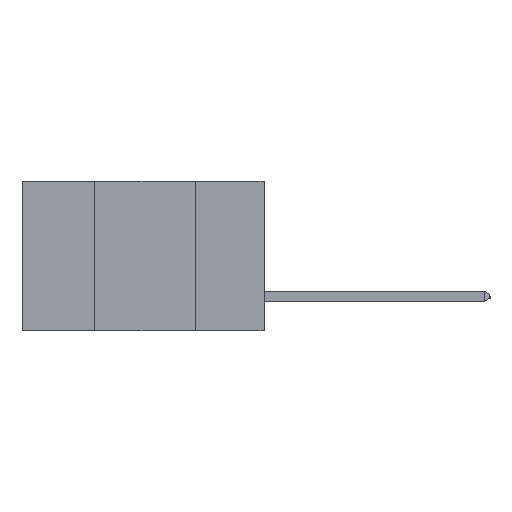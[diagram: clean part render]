
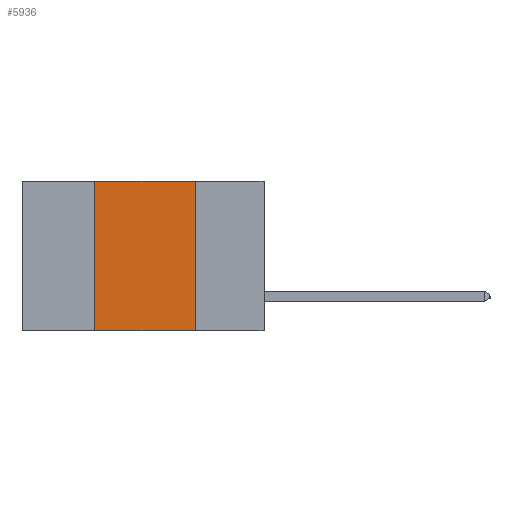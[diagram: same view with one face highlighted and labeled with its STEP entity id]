
A CAD part, left-side view. The second image highlights one B-rep face of the part: STEP entity #5936.
In plain terms, the highlighted planar face has unit normal (-1, 0, 0).
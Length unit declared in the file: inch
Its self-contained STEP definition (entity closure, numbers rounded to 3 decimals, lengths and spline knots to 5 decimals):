
#427 = CARTESIAN_POINT ( 'NONE',  ( 0., 0.42, -0.37 ) ) ;
#438 = VECTOR ( 'NONE', #7719, 39.37008 ) ;
#1325 = CARTESIAN_POINT ( 'NONE',  ( 0., 0.6, 0. ) ) ;
#1400 = ORIENTED_EDGE ( 'NONE', *, *, #5030, .F. ) ;
#1433 = ORIENTED_EDGE ( 'NONE', *, *, #4392, .F. ) ;
#1859 = FACE_OUTER_BOUND ( 'NONE', #6535, .T. ) ;
#2053 = VERTEX_POINT ( 'NONE', #9306 ) ;
#2086 = ORIENTED_EDGE ( 'NONE', *, *, #10315, .T. ) ;
#2499 = CARTESIAN_POINT ( 'NONE',  ( 0., 0.6, 0. ) ) ;
#3251 = DIRECTION ( 'NONE',  ( 0., 0., 1. ) ) ;
#3254 = CARTESIAN_POINT ( 'NONE',  ( 0., 0.42, 0. ) ) ;
#3283 = EDGE_CURVE ( 'NONE', #7934, #3319, #8841, .T. ) ;
#3319 = VERTEX_POINT ( 'NONE', #8916 ) ;
#3467 = DIRECTION ( 'NONE',  ( 1., 0., 0. ) ) ;
#4392 = EDGE_CURVE ( 'NONE', #2053, #7729, #8712, .T. ) ;
#4463 = CARTESIAN_POINT ( 'NONE',  ( 0., 0.17, -0.37 ) ) ;
#4879 = VECTOR ( 'NONE', #3251, 39.37008 ) ;
#5030 = EDGE_CURVE ( 'NONE', #3319, #2053, #8929, .T. ) ;
#5333 = PLANE ( 'NONE',  #9651 ) ;
#5475 = CARTESIAN_POINT ( 'NONE',  ( 0., 0.6, -0.37 ) ) ;
#5936 = ADVANCED_FACE ( 'NONE', ( #1859 ), #5333, .F. ) ;
#6320 = DIRECTION ( 'NONE',  ( 0., -1., 0. ) ) ;
#6535 = EDGE_LOOP ( 'NONE', ( #1433, #1400, #8598, #2086 ) ) ;
#7719 = DIRECTION ( 'NONE',  ( 0., -1., 0. ) ) ;
#7729 = VERTEX_POINT ( 'NONE', #4463 ) ;
#7934 = VERTEX_POINT ( 'NONE', #427 ) ;
#8313 = LINE ( 'NONE', #5475, #10016 ) ;
#8598 = ORIENTED_EDGE ( 'NONE', *, *, #3283, .F. ) ;
#8712 = LINE ( 'NONE', #10352, #10399 ) ;
#8841 = LINE ( 'NONE', #3254, #4879 ) ;
#8916 = CARTESIAN_POINT ( 'NONE',  ( 0., 0.42, 0. ) ) ;
#8929 = LINE ( 'NONE', #2499, #438 ) ;
#9306 = CARTESIAN_POINT ( 'NONE',  ( 0., 0.17, 0. ) ) ;
#9446 = DIRECTION ( 'NONE',  ( 0., 0., -1. ) ) ;
#9651 = AXIS2_PLACEMENT_3D ( 'NONE', #1325, #3467, #9659 ) ;
#9659 = DIRECTION ( 'NONE',  ( 0., 0., -1. ) ) ;
#10016 = VECTOR ( 'NONE', #6320, 39.37008 ) ;
#10315 = EDGE_CURVE ( 'NONE', #7934, #7729, #8313, .T. ) ;
#10352 = CARTESIAN_POINT ( 'NONE',  ( 0., 0.17, 0. ) ) ;
#10399 = VECTOR ( 'NONE', #9446, 39.37008 ) ;
